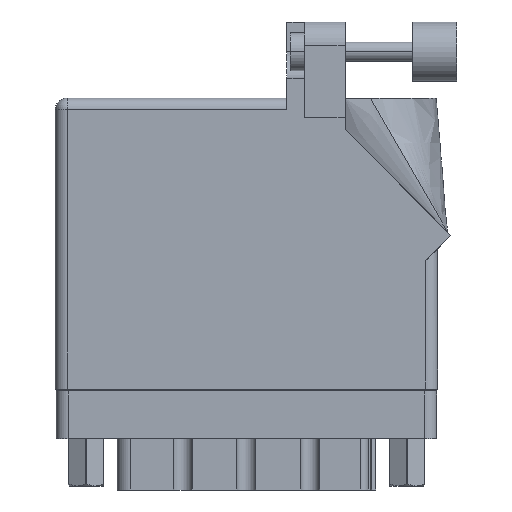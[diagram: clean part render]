
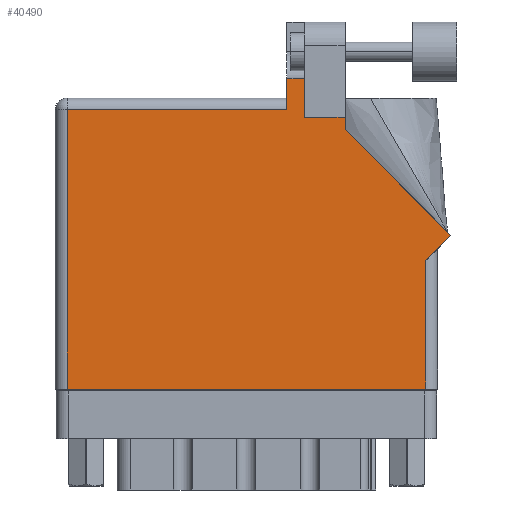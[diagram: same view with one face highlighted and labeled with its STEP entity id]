
A CAD part, front view. The second image highlights one B-rep face of the part: STEP entity #40490.
In plain terms, the highlighted face is planar.
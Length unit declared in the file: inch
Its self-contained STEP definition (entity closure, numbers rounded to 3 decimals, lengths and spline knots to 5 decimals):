
#358 = VECTOR ( 'NONE', #44579, 39.37008 ) ;
#1612 = CARTESIAN_POINT ( 'NONE',  ( 2.01, 0.737, 0. ) ) ;
#2740 = DIRECTION ( 'NONE',  ( -1., 0., 0. ) ) ;
#2846 = VECTOR ( 'NONE', #31572, 39.37008 ) ;
#4371 = CARTESIAN_POINT ( 'NONE',  ( 1.948, 0.737, 0. ) ) ;
#4597 = ORIENTED_EDGE ( 'NONE', *, *, #47521, .T. ) ;
#4844 = DIRECTION ( 'NONE',  ( -1., 0., 0. ) ) ;
#5352 = ORIENTED_EDGE ( 'NONE', *, *, #32768, .T. ) ;
#5457 = EDGE_CURVE ( 'NONE', #21050, #14009, #37073, .T. ) ;
#6791 = VECTOR ( 'NONE', #20481, 39.37008 ) ;
#6874 = VERTEX_POINT ( 'NONE', #33344 ) ;
#7020 = ORIENTED_EDGE ( 'NONE', *, *, #32003, .T. ) ;
#7335 = VERTEX_POINT ( 'NONE', #45469 ) ;
#7364 = DIRECTION ( 'NONE',  ( 0., -1., 0. ) ) ;
#7395 = EDGE_CURVE ( 'NONE', #38955, #21050, #8430, .T. ) ;
#7878 = DIRECTION ( 'NONE',  ( -0.707, 0.707, 0. ) ) ;
#8430 = LINE ( 'NONE', #18028, #20002 ) ;
#8678 = CARTESIAN_POINT ( 'NONE',  ( 0.062, 1.468, 0. ) ) ;
#8955 = ORIENTED_EDGE ( 'NONE', *, *, #23196, .T. ) ;
#9045 = CARTESIAN_POINT ( 'NONE',  ( 1.217, 1.468, 0. ) ) ;
#9219 = CARTESIAN_POINT ( 'NONE',  ( 1.217, 1.6315, 0. ) ) ;
#9636 = VECTOR ( 'NONE', #18420, 39.37008 ) ;
#9703 = DIRECTION ( 'NONE',  ( 0., -1., 0. ) ) ;
#10044 = VERTEX_POINT ( 'NONE', #15775 ) ;
#10227 = FACE_OUTER_BOUND ( 'NONE', #42889, .T. ) ;
#10480 = LINE ( 'NONE', #1612, #6791 ) ;
#10696 = LINE ( 'NONE', #14238, #358 ) ;
#11424 = LINE ( 'NONE', #18757, #9636 ) ;
#11959 = VECTOR ( 'NONE', #13329, 39.37008 ) ;
#12833 = VECTOR ( 'NONE', #9703, 39.37008 ) ;
#13058 = EDGE_CURVE ( 'NONE', #38449, #38955, #43075, .T. ) ;
#13329 = DIRECTION ( 'NONE',  ( -1., 0., 0. ) ) ;
#14009 = VERTEX_POINT ( 'NONE', #9045 ) ;
#14238 = CARTESIAN_POINT ( 'NONE',  ( 0., 0., 0. ) ) ;
#14388 = LINE ( 'NONE', #4371, #2846 ) ;
#15775 = CARTESIAN_POINT ( 'NONE',  ( 1.948, 0., 0. ) ) ;
#16099 = ORIENTED_EDGE ( 'NONE', *, *, #7395, .T. ) ;
#16560 = VERTEX_POINT ( 'NONE', #45533 ) ;
#18028 = CARTESIAN_POINT ( 'NONE',  ( 1.64177, 1.6315, 0. ) ) ;
#18420 = DIRECTION ( 'NONE',  ( 0., 1., 0. ) ) ;
#18757 = CARTESIAN_POINT ( 'NONE',  ( 1.524, 1.36442, 0. ) ) ;
#18851 = DIRECTION ( 'NONE',  ( 0., 0., -1. ) ) ;
#19124 = DIRECTION ( 'NONE',  ( 0., 1., 0. ) ) ;
#20002 = VECTOR ( 'NONE', #2740, 39.37008 ) ;
#20481 = DIRECTION ( 'NONE',  ( 0.707, 0.707, 0. ) ) ;
#21050 = VERTEX_POINT ( 'NONE', #9219 ) ;
#22587 = CARTESIAN_POINT ( 'NONE',  ( 0., 1.53, 0. ) ) ;
#22911 = PLANE ( 'NONE',  #34842 ) ;
#23045 = LINE ( 'NONE', #35528, #39999 ) ;
#23196 = EDGE_CURVE ( 'NONE', #41587, #24760, #49079, .T. ) ;
#24760 = VERTEX_POINT ( 'NONE', #43916 ) ;
#25049 = CARTESIAN_POINT ( 'NONE',  ( 1.524, 1.43, 0. ) ) ;
#26707 = VECTOR ( 'NONE', #7364, 39.37008 ) ;
#27370 = EDGE_CURVE ( 'NONE', #7335, #28617, #11424, .T. ) ;
#27980 = EDGE_CURVE ( 'NONE', #10044, #6874, #14388, .T. ) ;
#28617 = VERTEX_POINT ( 'NONE', #25049 ) ;
#31572 = DIRECTION ( 'NONE',  ( 0., 1., 0. ) ) ;
#32003 = EDGE_CURVE ( 'NONE', #14009, #41587, #41389, .T. ) ;
#32058 = CARTESIAN_POINT ( 'NONE',  ( 0., 1.468, 0. ) ) ;
#32208 = CARTESIAN_POINT ( 'NONE',  ( 1.311, 1.6315, 0. ) ) ;
#32335 = VECTOR ( 'NONE', #4844, 39.37008 ) ;
#32768 = EDGE_CURVE ( 'NONE', #24760, #10044, #10696, .T. ) ;
#32925 = CARTESIAN_POINT ( 'NONE',  ( 1.217, 1.53, 0. ) ) ;
#33147 = CARTESIAN_POINT ( 'NONE',  ( 1.524, 1.43, 0. ) ) ;
#33344 = CARTESIAN_POINT ( 'NONE',  ( 1.948, 0.675, 0. ) ) ;
#34842 = AXIS2_PLACEMENT_3D ( 'NONE', #22587, #18851, #49816 ) ;
#35528 = CARTESIAN_POINT ( 'NONE',  ( 2.08071, 0.80771, 0. ) ) ;
#37073 = LINE ( 'NONE', #32925, #12833 ) ;
#38449 = VERTEX_POINT ( 'NONE', #46156 ) ;
#38955 = VERTEX_POINT ( 'NONE', #32208 ) ;
#39665 = EDGE_CURVE ( 'NONE', #28617, #38449, #42259, .T. ) ;
#39999 = VECTOR ( 'NONE', #7878, 39.37008 ) ;
#40071 = VECTOR ( 'NONE', #19124, 39.37008 ) ;
#40490 = ADVANCED_FACE ( 'NONE', ( #10227 ), #22911, .F. ) ;
#40887 = ORIENTED_EDGE ( 'NONE', *, *, #27980, .T. ) ;
#41389 = LINE ( 'NONE', #32058, #32335 ) ;
#41587 = VERTEX_POINT ( 'NONE', #8678 ) ;
#41928 = ORIENTED_EDGE ( 'NONE', *, *, #5457, .T. ) ;
#42259 = LINE ( 'NONE', #33147, #11959 ) ;
#42309 = CARTESIAN_POINT ( 'NONE',  ( 0.062, 0., 0. ) ) ;
#42889 = EDGE_LOOP ( 'NONE', ( #45321, #16099, #41928, #7020, #8955, #5352, #40887, #48311, #4597, #46737, #46917 ) ) ;
#43075 = LINE ( 'NONE', #46527, #40071 ) ;
#43916 = CARTESIAN_POINT ( 'NONE',  ( 0.062, 0., 0. ) ) ;
#44579 = DIRECTION ( 'NONE',  ( 1., 0., 0. ) ) ;
#44627 = EDGE_CURVE ( 'NONE', #6874, #16560, #10480, .T. ) ;
#45321 = ORIENTED_EDGE ( 'NONE', *, *, #13058, .T. ) ;
#45469 = CARTESIAN_POINT ( 'NONE',  ( 1.524, 1.36442, 0. ) ) ;
#45533 = CARTESIAN_POINT ( 'NONE',  ( 2.08071, 0.80771, 0. ) ) ;
#46156 = CARTESIAN_POINT ( 'NONE',  ( 1.311, 1.43, 0. ) ) ;
#46527 = CARTESIAN_POINT ( 'NONE',  ( 1.311, 1.43, 0. ) ) ;
#46737 = ORIENTED_EDGE ( 'NONE', *, *, #27370, .T. ) ;
#46917 = ORIENTED_EDGE ( 'NONE', *, *, #39665, .T. ) ;
#47521 = EDGE_CURVE ( 'NONE', #16560, #7335, #23045, .T. ) ;
#48311 = ORIENTED_EDGE ( 'NONE', *, *, #44627, .T. ) ;
#49079 = LINE ( 'NONE', #42309, #26707 ) ;
#49816 = DIRECTION ( 'NONE',  ( -1., 0., 0. ) ) ;
